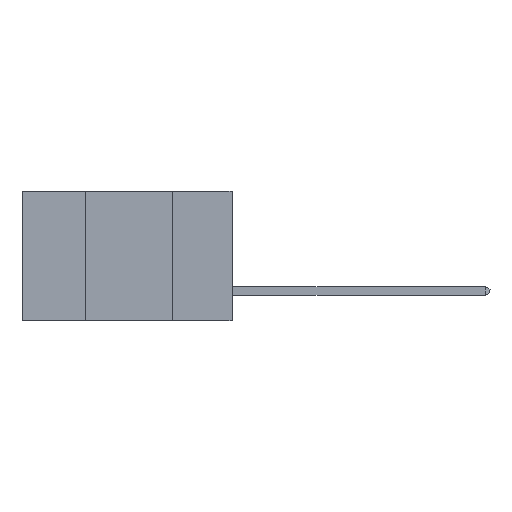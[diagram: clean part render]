
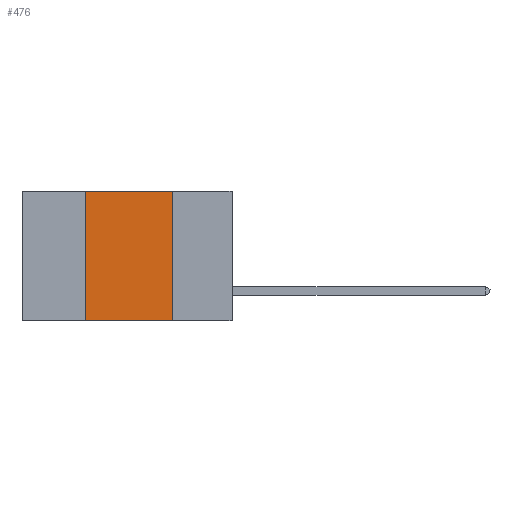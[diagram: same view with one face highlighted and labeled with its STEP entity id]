
A CAD part, left-side view. The second image highlights one B-rep face of the part: STEP entity #476.
In plain terms, the highlighted planar face has unit normal (-1, 0, 0).
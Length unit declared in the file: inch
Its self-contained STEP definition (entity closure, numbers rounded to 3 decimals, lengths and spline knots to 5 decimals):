
#476 = ADVANCED_FACE ( 'NONE', ( #4840 ), #5155, .F. ) ;
#533 = DIRECTION ( 'NONE',  ( 0., 0., -1. ) ) ;
#971 = CARTESIAN_POINT ( 'NONE',  ( 0., 0.17, 0. ) ) ;
#1663 = LINE ( 'NONE', #7906, #4044 ) ;
#1931 = CARTESIAN_POINT ( 'NONE',  ( 0., 0.42, -0.37 ) ) ;
#1958 = LINE ( 'NONE', #11160, #13959 ) ;
#3071 = EDGE_CURVE ( 'NONE', #4883, #14520, #1663, .T. ) ;
#3335 = AXIS2_PLACEMENT_3D ( 'NONE', #7545, #7492, #533 ) ;
#4033 = CARTESIAN_POINT ( 'NONE',  ( 0., 0.42, 0. ) ) ;
#4044 = VECTOR ( 'NONE', #14660, 39.37008 ) ;
#4158 = LINE ( 'NONE', #11340, #12841 ) ;
#4471 = LINE ( 'NONE', #5057, #9910 ) ;
#4840 = FACE_OUTER_BOUND ( 'NONE', #8010, .T. ) ;
#4883 = VERTEX_POINT ( 'NONE', #971 ) ;
#5057 = CARTESIAN_POINT ( 'NONE',  ( 0., 0.42, 0. ) ) ;
#5155 = PLANE ( 'NONE',  #3335 ) ;
#5831 = ORIENTED_EDGE ( 'NONE', *, *, #3071, .F. ) ;
#6515 = ORIENTED_EDGE ( 'NONE', *, *, #15086, .F. ) ;
#6873 = VERTEX_POINT ( 'NONE', #1931 ) ;
#7492 = DIRECTION ( 'NONE',  ( 1., 0., 0. ) ) ;
#7532 = DIRECTION ( 'NONE',  ( 0., -1., 0. ) ) ;
#7545 = CARTESIAN_POINT ( 'NONE',  ( 0., 0.6, 0. ) ) ;
#7710 = DIRECTION ( 'NONE',  ( 0., -1., 0. ) ) ;
#7906 = CARTESIAN_POINT ( 'NONE',  ( 0., 0.17, 0. ) ) ;
#8010 = EDGE_LOOP ( 'NONE', ( #5831, #6515, #11753, #10083 ) ) ;
#8903 = CARTESIAN_POINT ( 'NONE',  ( 0., 0.17, -0.37 ) ) ;
#9910 = VECTOR ( 'NONE', #11830, 39.37008 ) ;
#10083 = ORIENTED_EDGE ( 'NONE', *, *, #11986, .T. ) ;
#11160 = CARTESIAN_POINT ( 'NONE',  ( 0., 0.6, -0.37 ) ) ;
#11340 = CARTESIAN_POINT ( 'NONE',  ( 0., 0.6, 0. ) ) ;
#11753 = ORIENTED_EDGE ( 'NONE', *, *, #13746, .F. ) ;
#11830 = DIRECTION ( 'NONE',  ( 0., 0., 1. ) ) ;
#11986 = EDGE_CURVE ( 'NONE', #6873, #14520, #1958, .T. ) ;
#11992 = VERTEX_POINT ( 'NONE', #4033 ) ;
#12841 = VECTOR ( 'NONE', #7710, 39.37008 ) ;
#13746 = EDGE_CURVE ( 'NONE', #6873, #11992, #4471, .T. ) ;
#13959 = VECTOR ( 'NONE', #7532, 39.37008 ) ;
#14520 = VERTEX_POINT ( 'NONE', #8903 ) ;
#14660 = DIRECTION ( 'NONE',  ( 0., 0., -1. ) ) ;
#15086 = EDGE_CURVE ( 'NONE', #11992, #4883, #4158, .T. ) ;
